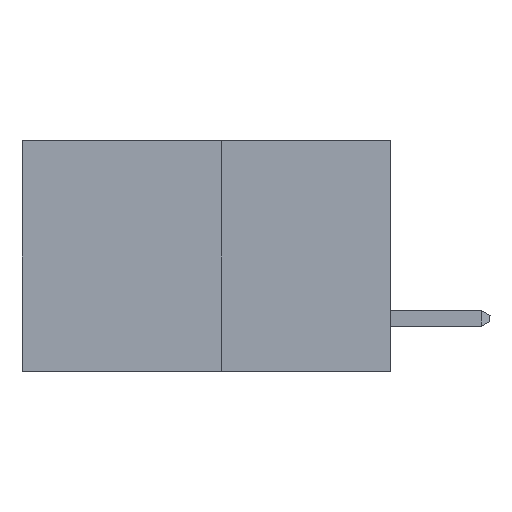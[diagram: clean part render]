
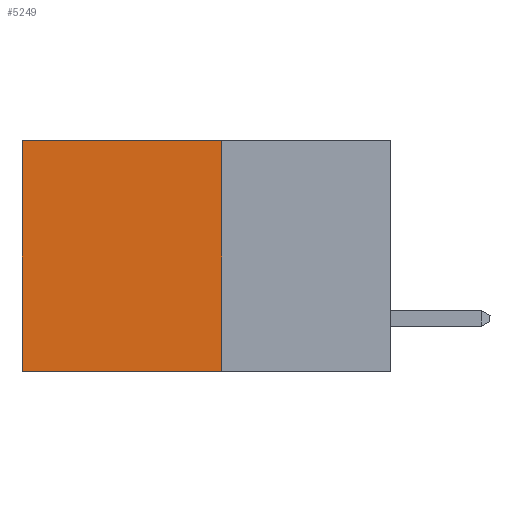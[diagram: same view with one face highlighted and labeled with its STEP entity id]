
A CAD part, left-side view. The second image highlights one B-rep face of the part: STEP entity #5249.
In plain terms, the highlighted planar face has unit normal (-1, 0, 0).
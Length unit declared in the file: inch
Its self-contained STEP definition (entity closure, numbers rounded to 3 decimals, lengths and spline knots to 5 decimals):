
#712 = EDGE_CURVE ( 'NONE', #4864, #2680, #2145, .T. ) ;
#1433 = CARTESIAN_POINT ( 'NONE',  ( 0.277, 0.27, -0.37 ) ) ;
#1731 = ORIENTED_EDGE ( 'NONE', *, *, #9162, .T. ) ;
#2145 = LINE ( 'NONE', #1433, #7319 ) ;
#2262 = CARTESIAN_POINT ( 'NONE',  ( 0.277, 0.27, -0.37 ) ) ;
#2680 = VERTEX_POINT ( 'NONE', #10174 ) ;
#3399 = CARTESIAN_POINT ( 'NONE',  ( 0.277, 0.27, 0. ) ) ;
#3874 = CARTESIAN_POINT ( 'NONE',  ( 0.277, 0.27, 0. ) ) ;
#4748 = CARTESIAN_POINT ( 'NONE',  ( 0.277, 0.59, 0. ) ) ;
#4821 = AXIS2_PLACEMENT_3D ( 'NONE', #9663, #8290, #8261 ) ;
#4864 = VERTEX_POINT ( 'NONE', #3399 ) ;
#4932 = DIRECTION ( 'NONE',  ( 0., 0., -1. ) ) ;
#5249 = ADVANCED_FACE ( 'NONE', ( #9720 ), #8361, .F. ) ;
#5355 = ORIENTED_EDGE ( 'NONE', *, *, #10348, .T. ) ;
#6119 = DIRECTION ( 'NONE',  ( 0., 0., -1. ) ) ;
#7212 = VECTOR ( 'NONE', #11395, 39.37008 ) ;
#7319 = VECTOR ( 'NONE', #6119, 39.37008 ) ;
#7551 = ORIENTED_EDGE ( 'NONE', *, *, #712, .F. ) ;
#7597 = LINE ( 'NONE', #2262, #12212 ) ;
#8191 = EDGE_LOOP ( 'NONE', ( #1731, #9186, #7551, #5355 ) ) ;
#8261 = DIRECTION ( 'NONE',  ( 0., 0., -1. ) ) ;
#8290 = DIRECTION ( 'NONE',  ( 1., 0., 0. ) ) ;
#8361 = PLANE ( 'NONE',  #4821 ) ;
#8637 = CARTESIAN_POINT ( 'NONE',  ( 0.277, 0.59, -0.37 ) ) ;
#8709 = EDGE_CURVE ( 'NONE', #2680, #9113, #7597, .T. ) ;
#9113 = VERTEX_POINT ( 'NONE', #8637 ) ;
#9150 = VECTOR ( 'NONE', #4932, 39.37008 ) ;
#9162 = EDGE_CURVE ( 'NONE', #9555, #9113, #9433, .T. ) ;
#9186 = ORIENTED_EDGE ( 'NONE', *, *, #8709, .F. ) ;
#9433 = LINE ( 'NONE', #12425, #9150 ) ;
#9555 = VERTEX_POINT ( 'NONE', #4748 ) ;
#9663 = CARTESIAN_POINT ( 'NONE',  ( 0.277, 0.27, -0.37 ) ) ;
#9720 = FACE_OUTER_BOUND ( 'NONE', #8191, .T. ) ;
#9980 = LINE ( 'NONE', #3874, #7212 ) ;
#10174 = CARTESIAN_POINT ( 'NONE',  ( 0.277, 0.27, -0.37 ) ) ;
#10348 = EDGE_CURVE ( 'NONE', #4864, #9555, #9980, .T. ) ;
#10826 = DIRECTION ( 'NONE',  ( 0., 1., 0. ) ) ;
#11395 = DIRECTION ( 'NONE',  ( 0., 1., 0. ) ) ;
#12212 = VECTOR ( 'NONE', #10826, 39.37008 ) ;
#12425 = CARTESIAN_POINT ( 'NONE',  ( 0.277, 0.59, -0.37 ) ) ;
